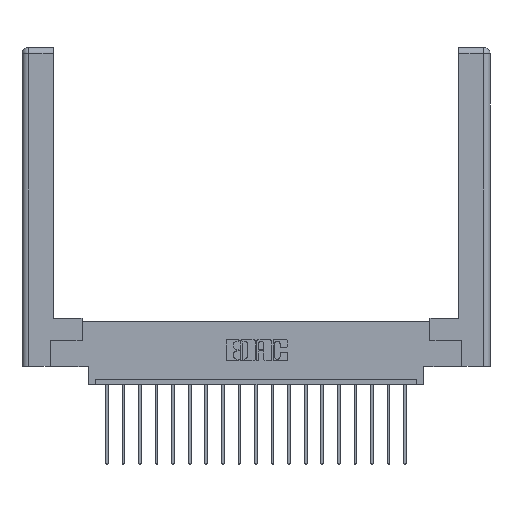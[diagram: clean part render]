
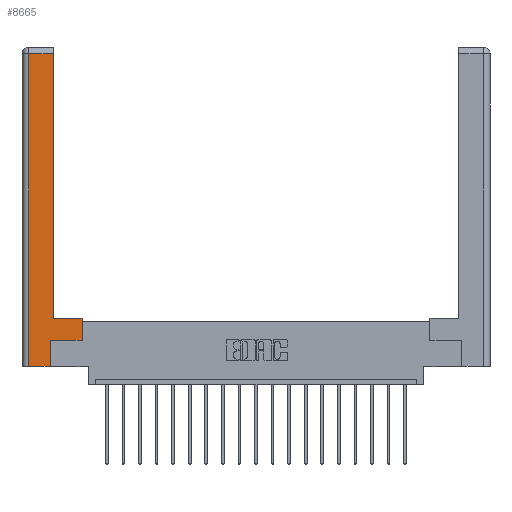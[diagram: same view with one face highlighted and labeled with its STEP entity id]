
A CAD part, top view. The second image highlights one B-rep face of the part: STEP entity #8665.
In plain terms, the highlighted planar face has unit normal (0, 0, 1).
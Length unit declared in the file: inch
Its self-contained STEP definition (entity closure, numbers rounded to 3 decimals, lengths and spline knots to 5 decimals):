
#434 = ORIENTED_EDGE ( 'NONE', *, *, #10159, .T. ) ;
#797 = VECTOR ( 'NONE', #18327, 39.37008 ) ;
#1123 = EDGE_CURVE ( 'NONE', #3281, #7392, #13328, .T. ) ;
#1198 = ORIENTED_EDGE ( 'NONE', *, *, #1123, .T. ) ;
#1530 = ORIENTED_EDGE ( 'NONE', *, *, #3799, .T. ) ;
#1679 = VERTEX_POINT ( 'NONE', #13811 ) ;
#2019 = CARTESIAN_POINT ( 'NONE',  ( 0.295, 0.45, 0. ) ) ;
#2341 = CARTESIAN_POINT ( 'NONE',  ( 0.565, 0.45, 0. ) ) ;
#2466 = VERTEX_POINT ( 'NONE', #2555 ) ;
#2555 = CARTESIAN_POINT ( 'NONE',  ( 0.295, 0.45, 0. ) ) ;
#2767 = CARTESIAN_POINT ( 'NONE',  ( 0.265, 0., 0. ) ) ;
#3281 = VERTEX_POINT ( 'NONE', #18508 ) ;
#3370 = LINE ( 'NONE', #12045, #17307 ) ;
#3756 = LINE ( 'NONE', #8826, #5187 ) ;
#3799 = EDGE_CURVE ( 'NONE', #2466, #6237, #3370, .T. ) ;
#3846 = CARTESIAN_POINT ( 'NONE',  ( 0.565, 0.45, 0. ) ) ;
#4405 = LINE ( 'NONE', #6033, #797 ) ;
#5187 = VECTOR ( 'NONE', #7485, 39.37008 ) ;
#6033 = CARTESIAN_POINT ( 'NONE',  ( 0.565, 0.245, 0. ) ) ;
#6237 = VERTEX_POINT ( 'NONE', #8263 ) ;
#6271 = CARTESIAN_POINT ( 'NONE',  ( 0., 0., 0. ) ) ;
#6379 = EDGE_CURVE ( 'NONE', #1679, #19473, #4405, .T. ) ;
#6937 = LINE ( 'NONE', #14531, #8137 ) ;
#7392 = VERTEX_POINT ( 'NONE', #17047 ) ;
#7485 = DIRECTION ( 'NONE',  ( 1., 0., 0. ) ) ;
#7536 = EDGE_CURVE ( 'NONE', #19473, #19379, #14718, .T. ) ;
#8137 = VECTOR ( 'NONE', #8172, 39.37008 ) ;
#8172 = DIRECTION ( 'NONE',  ( 0., 1., 0. ) ) ;
#8263 = CARTESIAN_POINT ( 'NONE',  ( 0.295, 2.94, 0. ) ) ;
#8665 = ADVANCED_FACE ( 'NONE', ( #15118 ), #10705, .F. ) ;
#8826 = CARTESIAN_POINT ( 'NONE',  ( 0.265, 0., 0. ) ) ;
#10126 = VECTOR ( 'NONE', #11617, 39.37008 ) ;
#10159 = EDGE_CURVE ( 'NONE', #18541, #1679, #6937, .T. ) ;
#10705 = PLANE ( 'NONE',  #11293 ) ;
#10982 = DIRECTION ( 'NONE',  ( 0., 0., -1. ) ) ;
#11025 = CARTESIAN_POINT ( 'NONE',  ( 0.0615, 2.94, 0. ) ) ;
#11191 = VECTOR ( 'NONE', #11789, 39.37008 ) ;
#11293 = AXIS2_PLACEMENT_3D ( 'NONE', #6271, #10982, #18480 ) ;
#11617 = DIRECTION ( 'NONE',  ( 0., 1., 0. ) ) ;
#11789 = DIRECTION ( 'NONE',  ( 0., -1., 0. ) ) ;
#11918 = EDGE_CURVE ( 'NONE', #7392, #18541, #3756, .T. ) ;
#11973 = EDGE_LOOP ( 'NONE', ( #1530, #19270, #1198, #18914, #434, #18860, #15960, #17011 ) ) ;
#11995 = LINE ( 'NONE', #2019, #18717 ) ;
#12045 = CARTESIAN_POINT ( 'NONE',  ( 0.295, 3., 0. ) ) ;
#13197 = CARTESIAN_POINT ( 'NONE',  ( 0.0615, 0., 0. ) ) ;
#13328 = LINE ( 'NONE', #13197, #11191 ) ;
#13361 = VECTOR ( 'NONE', #13913, 39.37008 ) ;
#13811 = CARTESIAN_POINT ( 'NONE',  ( 0.265, 0.245, 0. ) ) ;
#13913 = DIRECTION ( 'NONE',  ( -1., 0., 0. ) ) ;
#14182 = DIRECTION ( 'NONE',  ( -1., 0., 0. ) ) ;
#14531 = CARTESIAN_POINT ( 'NONE',  ( 0.265, 0.245, 0. ) ) ;
#14718 = LINE ( 'NONE', #3846, #10126 ) ;
#15118 = FACE_OUTER_BOUND ( 'NONE', #11973, .T. ) ;
#15960 = ORIENTED_EDGE ( 'NONE', *, *, #7536, .T. ) ;
#16304 = EDGE_CURVE ( 'NONE', #6237, #3281, #18409, .T. ) ;
#16569 = DIRECTION ( 'NONE',  ( 0., 1., 0. ) ) ;
#17011 = ORIENTED_EDGE ( 'NONE', *, *, #19195, .T. ) ;
#17047 = CARTESIAN_POINT ( 'NONE',  ( 0.0615, 0., 0. ) ) ;
#17307 = VECTOR ( 'NONE', #16569, 39.37008 ) ;
#17924 = CARTESIAN_POINT ( 'NONE',  ( 0.565, 0.245, 0. ) ) ;
#18327 = DIRECTION ( 'NONE',  ( 1., 0., 0. ) ) ;
#18409 = LINE ( 'NONE', #11025, #13361 ) ;
#18480 = DIRECTION ( 'NONE',  ( -1., 0., 0. ) ) ;
#18508 = CARTESIAN_POINT ( 'NONE',  ( 0.0615, 2.94, 0. ) ) ;
#18541 = VERTEX_POINT ( 'NONE', #2767 ) ;
#18717 = VECTOR ( 'NONE', #14182, 39.37008 ) ;
#18860 = ORIENTED_EDGE ( 'NONE', *, *, #6379, .T. ) ;
#18914 = ORIENTED_EDGE ( 'NONE', *, *, #11918, .T. ) ;
#19195 = EDGE_CURVE ( 'NONE', #19379, #2466, #11995, .T. ) ;
#19270 = ORIENTED_EDGE ( 'NONE', *, *, #16304, .T. ) ;
#19379 = VERTEX_POINT ( 'NONE', #2341 ) ;
#19473 = VERTEX_POINT ( 'NONE', #17924 ) ;
